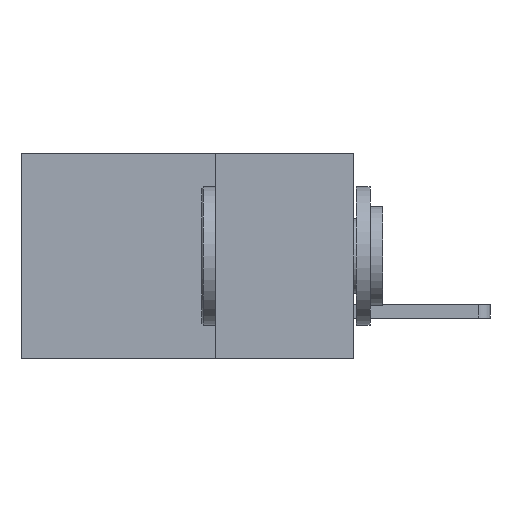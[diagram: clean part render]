
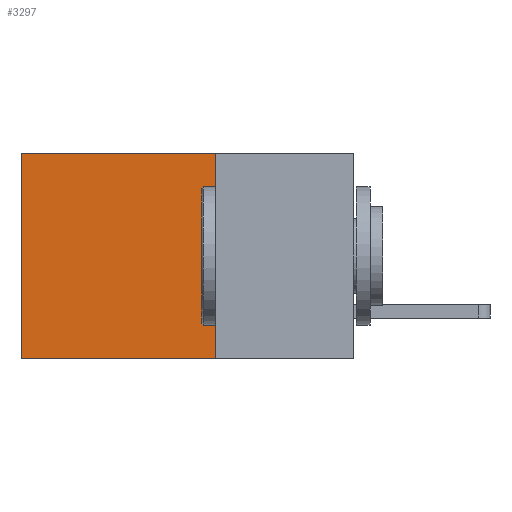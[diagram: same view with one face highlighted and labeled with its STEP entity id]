
A CAD part, left-side view. The second image highlights one B-rep face of the part: STEP entity #3297.
In plain terms, the highlighted planar face has unit normal (-1, 0, 0).
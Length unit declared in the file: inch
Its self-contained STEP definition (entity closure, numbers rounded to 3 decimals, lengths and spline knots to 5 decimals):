
#175 = DIRECTION ( 'NONE',  ( 0., 0., -1. ) ) ;
#333 = CARTESIAN_POINT ( 'NONE',  ( 0.2875, 0.25, 0. ) ) ;
#879 = DIRECTION ( 'NONE',  ( 0., 0., -1. ) ) ;
#1616 = ORIENTED_EDGE ( 'NONE', *, *, #3454, .F. ) ;
#1641 = DIRECTION ( 'NONE',  ( 0., 1., 0. ) ) ;
#1865 = CARTESIAN_POINT ( 'NONE',  ( 0.2875, 0.25, -0.37 ) ) ;
#3297 = ADVANCED_FACE ( 'NONE', ( #4463 ), #5897, .F. ) ;
#3390 = LINE ( 'NONE', #8760, #5709 ) ;
#3454 = EDGE_CURVE ( 'NONE', #9041, #12669, #11525, .T. ) ;
#4088 = ORIENTED_EDGE ( 'NONE', *, *, #8849, .F. ) ;
#4463 = FACE_OUTER_BOUND ( 'NONE', #9160, .T. ) ;
#4734 = DIRECTION ( 'NONE',  ( 1., 0., 0. ) ) ;
#4981 = VERTEX_POINT ( 'NONE', #13873 ) ;
#5029 = CARTESIAN_POINT ( 'NONE',  ( 0.2875, 0.6, -0.37 ) ) ;
#5330 = AXIS2_PLACEMENT_3D ( 'NONE', #333, #4734, #8210 ) ;
#5709 = VECTOR ( 'NONE', #7798, 39.37008 ) ;
#5897 = PLANE ( 'NONE',  #5330 ) ;
#6097 = ORIENTED_EDGE ( 'NONE', *, *, #9590, .T. ) ;
#6870 = CARTESIAN_POINT ( 'NONE',  ( 0.2875, 0.6, 0. ) ) ;
#7798 = DIRECTION ( 'NONE',  ( 0., 1., 0. ) ) ;
#7874 = EDGE_CURVE ( 'NONE', #10659, #12669, #10832, .T. ) ;
#8210 = DIRECTION ( 'NONE',  ( 0., 0., -1. ) ) ;
#8760 = CARTESIAN_POINT ( 'NONE',  ( 0.2875, 0.25, 0. ) ) ;
#8799 = CARTESIAN_POINT ( 'NONE',  ( 0.2875, 0.6, 0. ) ) ;
#8849 = EDGE_CURVE ( 'NONE', #4981, #9041, #9858, .T. ) ;
#9041 = VERTEX_POINT ( 'NONE', #1865 ) ;
#9130 = ORIENTED_EDGE ( 'NONE', *, *, #7874, .T. ) ;
#9160 = EDGE_LOOP ( 'NONE', ( #9130, #1616, #4088, #6097 ) ) ;
#9367 = VECTOR ( 'NONE', #879, 39.37008 ) ;
#9590 = EDGE_CURVE ( 'NONE', #4981, #10659, #3390, .T. ) ;
#9858 = LINE ( 'NONE', #10064, #11245 ) ;
#10064 = CARTESIAN_POINT ( 'NONE',  ( 0.2875, 0.25, 0. ) ) ;
#10659 = VERTEX_POINT ( 'NONE', #6870 ) ;
#10832 = LINE ( 'NONE', #8799, #9367 ) ;
#10900 = VECTOR ( 'NONE', #1641, 39.37008 ) ;
#11245 = VECTOR ( 'NONE', #175, 39.37008 ) ;
#11457 = CARTESIAN_POINT ( 'NONE',  ( 0.2875, 0.25, -0.37 ) ) ;
#11525 = LINE ( 'NONE', #11457, #10900 ) ;
#12669 = VERTEX_POINT ( 'NONE', #5029 ) ;
#13873 = CARTESIAN_POINT ( 'NONE',  ( 0.2875, 0.25, 0. ) ) ;
